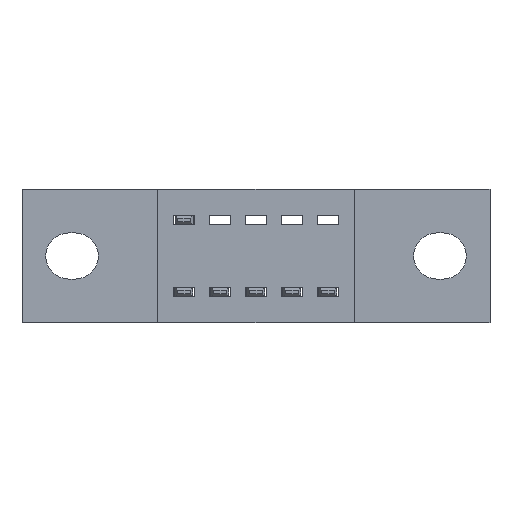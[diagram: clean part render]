
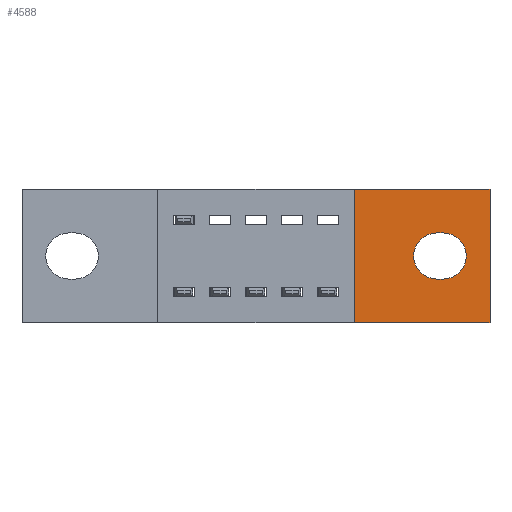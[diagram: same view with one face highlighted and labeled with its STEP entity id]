
A CAD part, front view. The second image highlights one B-rep face of the part: STEP entity #4588.
In plain terms, the highlighted planar face has unit normal (0, -1, 0).
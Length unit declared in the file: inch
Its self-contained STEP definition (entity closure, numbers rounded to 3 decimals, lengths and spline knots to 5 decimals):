
#9 = DIRECTION ( 'NONE',  ( 1., 0., 0. ) ) ;
#34 = CARTESIAN_POINT ( 'NONE',  ( 0.923, 0., -0.37 ) ) ;
#267 = EDGE_CURVE ( 'NONE', #6642, #3016, #6915, .T. ) ;
#496 = DIRECTION ( 'NONE',  ( 0., 0., 1. ) ) ;
#713 = VERTEX_POINT ( 'NONE', #4714 ) ;
#717 = LINE ( 'NONE', #7202, #2662 ) ;
#849 = ORIENTED_EDGE ( 'NONE', *, *, #7433, .T. ) ;
#865 = CARTESIAN_POINT ( 'NONE',  ( 1.17, 0., -0.185 ) ) ;
#913 = VERTEX_POINT ( 'NONE', #5801 ) ;
#916 = DIRECTION ( 'NONE',  ( -1., 0., 0. ) ) ;
#1042 = CARTESIAN_POINT ( 'NONE',  ( 0., 0., -0.37 ) ) ;
#1062 = PLANE ( 'NONE',  #4977 ) ;
#1065 = ORIENTED_EDGE ( 'NONE', *, *, #3601, .F. ) ;
#1310 = CARTESIAN_POINT ( 'NONE',  ( 0., 0., 0. ) ) ;
#1515 = LINE ( 'NONE', #5746, #1929 ) ;
#1533 = DIRECTION ( 'NONE',  ( 0., 0., -1. ) ) ;
#1573 = DIRECTION ( 'NONE',  ( 1., 0., 0. ) ) ;
#1614 = LINE ( 'NONE', #6292, #5995 ) ;
#1640 = EDGE_LOOP ( 'NONE', ( #1065, #2773, #4375, #5891 ) ) ;
#1673 = CARTESIAN_POINT ( 'NONE',  ( 1.152, 0., -0.185 ) ) ;
#1749 = EDGE_CURVE ( 'NONE', #3016, #4015, #1614, .T. ) ;
#1804 = DIRECTION ( 'NONE',  ( 0., 0., -1. ) ) ;
#1816 = DIRECTION ( 'NONE',  ( 0., -1., 0. ) ) ;
#1929 = VECTOR ( 'NONE', #5742, 39.37008 ) ;
#2087 = EDGE_CURVE ( 'NONE', #2652, #4541, #1515, .T. ) ;
#2109 = FACE_BOUND ( 'NONE', #6124, .T. ) ;
#2334 = DIRECTION ( 'NONE',  ( 0., 0., -1. ) ) ;
#2342 = AXIS2_PLACEMENT_3D ( 'NONE', #1673, #5866, #2334 ) ;
#2480 = CIRCLE ( 'NONE', #2342, 0.064 ) ;
#2595 = ORIENTED_EDGE ( 'NONE', *, *, #2087, .T. ) ;
#2652 = VERTEX_POINT ( 'NONE', #4813 ) ;
#2662 = VECTOR ( 'NONE', #916, 39.37008 ) ;
#2742 = CARTESIAN_POINT ( 'NONE',  ( 1.152, 0., -0.249 ) ) ;
#2773 = ORIENTED_EDGE ( 'NONE', *, *, #7228, .F. ) ;
#2786 = VECTOR ( 'NONE', #496, 39.37008 ) ;
#2967 = LINE ( 'NONE', #34, #2786 ) ;
#3016 = VERTEX_POINT ( 'NONE', #5934 ) ;
#3601 = EDGE_CURVE ( 'NONE', #713, #6642, #2967, .T. ) ;
#3680 = CIRCLE ( 'NONE', #6928, 0.064 ) ;
#3775 = VERTEX_POINT ( 'NONE', #6492 ) ;
#4015 = VERTEX_POINT ( 'NONE', #4323 ) ;
#4157 = ORIENTED_EDGE ( 'NONE', *, *, #6471, .T. ) ;
#4323 = CARTESIAN_POINT ( 'NONE',  ( 1.3, 0., -0.37 ) ) ;
#4375 = ORIENTED_EDGE ( 'NONE', *, *, #1749, .F. ) ;
#4541 = VERTEX_POINT ( 'NONE', #2742 ) ;
#4588 = ADVANCED_FACE ( 'NONE', ( #2109, #6709 ), #1062, .T. ) ;
#4714 = CARTESIAN_POINT ( 'NONE',  ( 0.923, 0., -0.37 ) ) ;
#4813 = CARTESIAN_POINT ( 'NONE',  ( 1.17, 0., -0.249 ) ) ;
#4977 = AXIS2_PLACEMENT_3D ( 'NONE', #1042, #1816, #1804 ) ;
#5032 = VECTOR ( 'NONE', #1573, 39.37008 ) ;
#5213 = DIRECTION ( 'NONE',  ( 0., 1., 0. ) ) ;
#5376 = VECTOR ( 'NONE', #9, 39.37008 ) ;
#5742 = DIRECTION ( 'NONE',  ( -1., 0., 0. ) ) ;
#5746 = CARTESIAN_POINT ( 'NONE',  ( 1.17, 0., -0.249 ) ) ;
#5801 = CARTESIAN_POINT ( 'NONE',  ( 1.17, 0., -0.121 ) ) ;
#5820 = DIRECTION ( 'NONE',  ( 0., 0., -1. ) ) ;
#5866 = DIRECTION ( 'NONE',  ( 0., 1., 0. ) ) ;
#5891 = ORIENTED_EDGE ( 'NONE', *, *, #267, .F. ) ;
#5934 = CARTESIAN_POINT ( 'NONE',  ( 1.3, 0., 0. ) ) ;
#5995 = VECTOR ( 'NONE', #5820, 39.37008 ) ;
#6124 = EDGE_LOOP ( 'NONE', ( #849, #2595, #4157, #7096 ) ) ;
#6292 = CARTESIAN_POINT ( 'NONE',  ( 1.3, 0., 0. ) ) ;
#6350 = EDGE_CURVE ( 'NONE', #3775, #913, #7649, .T. ) ;
#6471 = EDGE_CURVE ( 'NONE', #4541, #3775, #2480, .T. ) ;
#6492 = CARTESIAN_POINT ( 'NONE',  ( 1.152, 0., -0.121 ) ) ;
#6642 = VERTEX_POINT ( 'NONE', #7520 ) ;
#6709 = FACE_OUTER_BOUND ( 'NONE', #1640, .T. ) ;
#6822 = CARTESIAN_POINT ( 'NONE',  ( 1.17, 0., -0.121 ) ) ;
#6915 = LINE ( 'NONE', #1310, #5376 ) ;
#6928 = AXIS2_PLACEMENT_3D ( 'NONE', #865, #5213, #1533 ) ;
#7096 = ORIENTED_EDGE ( 'NONE', *, *, #6350, .T. ) ;
#7202 = CARTESIAN_POINT ( 'NONE',  ( 0., 0., -0.37 ) ) ;
#7228 = EDGE_CURVE ( 'NONE', #4015, #713, #717, .T. ) ;
#7433 = EDGE_CURVE ( 'NONE', #913, #2652, #3680, .T. ) ;
#7520 = CARTESIAN_POINT ( 'NONE',  ( 0.923, 0., 0. ) ) ;
#7649 = LINE ( 'NONE', #6822, #5032 ) ;
